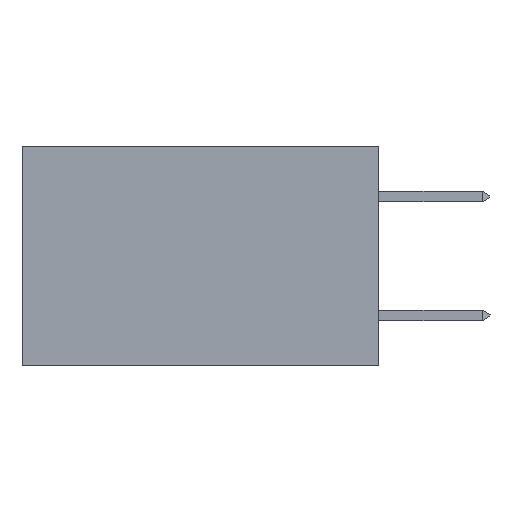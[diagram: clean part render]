
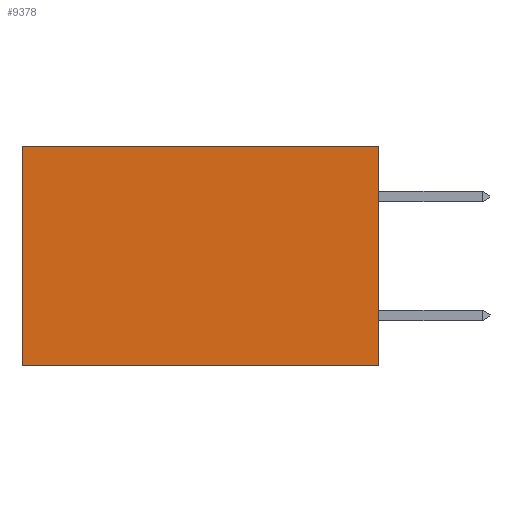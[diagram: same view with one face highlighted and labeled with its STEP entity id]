
A CAD part, left-side view. The second image highlights one B-rep face of the part: STEP entity #9378.
In plain terms, the highlighted planar face has unit normal (-1, 0, 0).
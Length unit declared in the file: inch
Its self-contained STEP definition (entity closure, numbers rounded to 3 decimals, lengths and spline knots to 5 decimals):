
#282 = CARTESIAN_POINT ( 'NONE',  ( 0.298, 0.6, 0. ) ) ;
#317 = VECTOR ( 'NONE', #5091, 39.37008 ) ;
#395 = VERTEX_POINT ( 'NONE', #8715 ) ;
#570 = LINE ( 'NONE', #2327, #3425 ) ;
#690 = DIRECTION ( 'NONE',  ( 0., 1., 0. ) ) ;
#968 = VERTEX_POINT ( 'NONE', #10824 ) ;
#1444 = EDGE_LOOP ( 'NONE', ( #2348, #2316, #10296, #3007 ) ) ;
#1567 = CARTESIAN_POINT ( 'NONE',  ( 0.298, 0., 0. ) ) ;
#1767 = VERTEX_POINT ( 'NONE', #7517 ) ;
#2316 = ORIENTED_EDGE ( 'NONE', *, *, #6707, .F. ) ;
#2327 = CARTESIAN_POINT ( 'NONE',  ( 0.298, 0., -0.37 ) ) ;
#2348 = ORIENTED_EDGE ( 'NONE', *, *, #4385, .T. ) ;
#2562 = VERTEX_POINT ( 'NONE', #10495 ) ;
#2942 = PLANE ( 'NONE',  #10753 ) ;
#3007 = ORIENTED_EDGE ( 'NONE', *, *, #7702, .T. ) ;
#3425 = VECTOR ( 'NONE', #10881, 39.37008 ) ;
#4385 = EDGE_CURVE ( 'NONE', #395, #968, #8550, .T. ) ;
#5091 = DIRECTION ( 'NONE',  ( 0., 0., -1. ) ) ;
#5340 = VECTOR ( 'NONE', #690, 39.37008 ) ;
#5645 = LINE ( 'NONE', #1567, #5340 ) ;
#5670 = CARTESIAN_POINT ( 'NONE',  ( 0.298, 0., 0. ) ) ;
#6121 = CARTESIAN_POINT ( 'NONE',  ( 0.298, 0., 0. ) ) ;
#6707 = EDGE_CURVE ( 'NONE', #1767, #968, #570, .T. ) ;
#7198 = LINE ( 'NONE', #6121, #11353 ) ;
#7517 = CARTESIAN_POINT ( 'NONE',  ( 0.298, 0., -0.37 ) ) ;
#7702 = EDGE_CURVE ( 'NONE', #2562, #395, #5645, .T. ) ;
#8550 = LINE ( 'NONE', #282, #317 ) ;
#8584 = DIRECTION ( 'NONE',  ( 1., 0., 0. ) ) ;
#8715 = CARTESIAN_POINT ( 'NONE',  ( 0.298, 0.6, 0. ) ) ;
#9378 = ADVANCED_FACE ( 'NONE', ( #9461 ), #2942, .F. ) ;
#9461 = FACE_OUTER_BOUND ( 'NONE', #1444, .T. ) ;
#9605 = DIRECTION ( 'NONE',  ( 0., 0., -1. ) ) ;
#10016 = DIRECTION ( 'NONE',  ( 0., 0., -1. ) ) ;
#10296 = ORIENTED_EDGE ( 'NONE', *, *, #11923, .F. ) ;
#10495 = CARTESIAN_POINT ( 'NONE',  ( 0.298, 0., 0. ) ) ;
#10753 = AXIS2_PLACEMENT_3D ( 'NONE', #5670, #8584, #9605 ) ;
#10824 = CARTESIAN_POINT ( 'NONE',  ( 0.298, 0.6, -0.37 ) ) ;
#10881 = DIRECTION ( 'NONE',  ( 0., 1., 0. ) ) ;
#11353 = VECTOR ( 'NONE', #10016, 39.37008 ) ;
#11923 = EDGE_CURVE ( 'NONE', #2562, #1767, #7198, .T. ) ;
